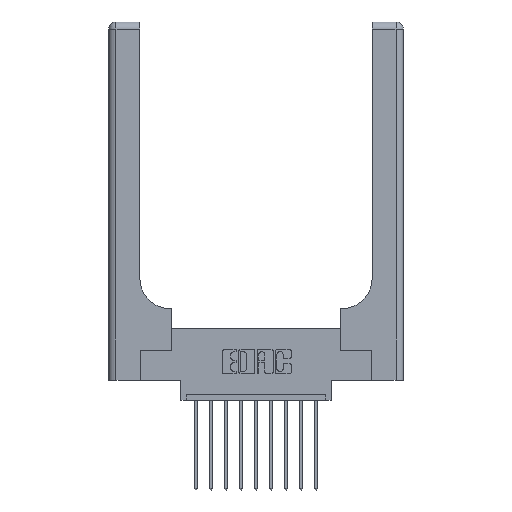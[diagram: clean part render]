
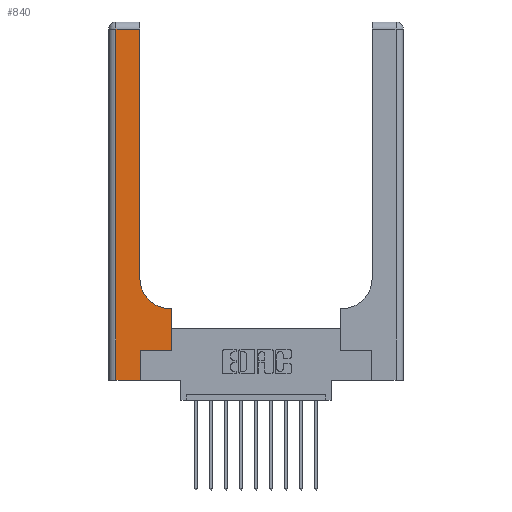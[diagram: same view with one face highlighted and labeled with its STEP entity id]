
A CAD part, top view. The second image highlights one B-rep face of the part: STEP entity #840.
In plain terms, the highlighted planar face has unit normal (0, 0, 1).
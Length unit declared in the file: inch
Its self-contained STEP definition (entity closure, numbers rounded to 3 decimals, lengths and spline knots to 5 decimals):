
#164 = VECTOR ( 'NONE', #4337, 39.37008 ) ;
#223 = EDGE_CURVE ( 'NONE', #14110, #13088, #5973, .T. ) ;
#840 = ADVANCED_FACE ( 'NONE', ( #7039 ), #7645, .F. ) ;
#1093 = VERTEX_POINT ( 'NONE', #11321 ) ;
#1422 = CARTESIAN_POINT ( 'NONE',  ( 0.51, 0.85, 0.37 ) ) ;
#1698 = EDGE_CURVE ( 'NONE', #5517, #12729, #12612, .T. ) ;
#1983 = EDGE_CURVE ( 'NONE', #14137, #7401, #2414, .T. ) ;
#1998 = DIRECTION ( 'NONE',  ( -1., 0., 0. ) ) ;
#2288 = VECTOR ( 'NONE', #9774, 39.37008 ) ;
#2414 = CIRCLE ( 'NONE', #3312, 0.25 ) ;
#2936 = VECTOR ( 'NONE', #14095, 39.37008 ) ;
#3136 = VERTEX_POINT ( 'NONE', #6033 ) ;
#3199 = VECTOR ( 'NONE', #10997, 39.37008 ) ;
#3218 = ORIENTED_EDGE ( 'NONE', *, *, #1983, .T. ) ;
#3287 = CARTESIAN_POINT ( 'NONE',  ( 0.26, 2.94, 0.37 ) ) ;
#3312 = AXIS2_PLACEMENT_3D ( 'NONE', #1422, #7130, #13097 ) ;
#3319 = ORIENTED_EDGE ( 'NONE', *, *, #223, .T. ) ;
#3345 = LINE ( 'NONE', #13888, #164 ) ;
#3554 = CARTESIAN_POINT ( 'NONE',  ( 0.51, 0.6, 0.37 ) ) ;
#3620 = EDGE_LOOP ( 'NONE', ( #14526, #9039, #9863, #4403, #15283, #3319, #12681, #5768, #3218 ) ) ;
#3802 = EDGE_CURVE ( 'NONE', #7401, #14683, #9755, .T. ) ;
#4337 = DIRECTION ( 'NONE',  ( 0., -1., 0. ) ) ;
#4403 = ORIENTED_EDGE ( 'NONE', *, *, #1698, .T. ) ;
#5284 = DIRECTION ( 'NONE',  ( -1., 0., 0. ) ) ;
#5517 = VERTEX_POINT ( 'NONE', #9015 ) ;
#5768 = ORIENTED_EDGE ( 'NONE', *, *, #8043, .T. ) ;
#5973 = LINE ( 'NONE', #12957, #14494 ) ;
#6033 = CARTESIAN_POINT ( 'NONE',  ( 0.528, 0.6, 0.37 ) ) ;
#6101 = CARTESIAN_POINT ( 'NONE',  ( 0.26, 0.85, 0.37 ) ) ;
#6198 = DIRECTION ( 'NONE',  ( 1., 0., 0. ) ) ;
#6939 = DIRECTION ( 'NONE',  ( 0., 1., 0. ) ) ;
#7039 = FACE_OUTER_BOUND ( 'NONE', #3620, .T. ) ;
#7130 = DIRECTION ( 'NONE',  ( 0., 0., -1. ) ) ;
#7401 = VERTEX_POINT ( 'NONE', #6101 ) ;
#7417 = VECTOR ( 'NONE', #6198, 39.37008 ) ;
#7645 = PLANE ( 'NONE',  #10521 ) ;
#7747 = DIRECTION ( 'NONE',  ( 0., 0., -1. ) ) ;
#8011 = LINE ( 'NONE', #10729, #2288 ) ;
#8043 = EDGE_CURVE ( 'NONE', #3136, #14137, #8011, .T. ) ;
#8693 = VECTOR ( 'NONE', #5284, 39.37008 ) ;
#9015 = CARTESIAN_POINT ( 'NONE',  ( 0.06, 0., 0.37 ) ) ;
#9039 = ORIENTED_EDGE ( 'NONE', *, *, #9614, .T. ) ;
#9614 = EDGE_CURVE ( 'NONE', #14683, #1093, #10550, .T. ) ;
#9755 = LINE ( 'NONE', #12920, #2936 ) ;
#9774 = DIRECTION ( 'NONE',  ( -1., 0., 0. ) ) ;
#9863 = ORIENTED_EDGE ( 'NONE', *, *, #15217, .T. ) ;
#10453 = CARTESIAN_POINT ( 'NONE',  ( 0.265, 0., 0.37 ) ) ;
#10521 = AXIS2_PLACEMENT_3D ( 'NONE', #14770, #7747, #1998 ) ;
#10550 = LINE ( 'NONE', #14643, #8693 ) ;
#10729 = CARTESIAN_POINT ( 'NONE',  ( 0.26, 0.6, 0.37 ) ) ;
#10834 = CARTESIAN_POINT ( 'NONE',  ( 0.528, 0.25, 0.37 ) ) ;
#10997 = DIRECTION ( 'NONE',  ( 0., 1., 0. ) ) ;
#11149 = LINE ( 'NONE', #10453, #14080 ) ;
#11321 = CARTESIAN_POINT ( 'NONE',  ( 0.06, 2.94, 0.37 ) ) ;
#11812 = DIRECTION ( 'NONE',  ( 1., 0., 0. ) ) ;
#12027 = CARTESIAN_POINT ( 'NONE',  ( 0.265, 0., 0.37 ) ) ;
#12612 = LINE ( 'NONE', #13285, #7417 ) ;
#12681 = ORIENTED_EDGE ( 'NONE', *, *, #14286, .T. ) ;
#12729 = VERTEX_POINT ( 'NONE', #12027 ) ;
#12920 = CARTESIAN_POINT ( 'NONE',  ( 0.26, 3., 0.37 ) ) ;
#12957 = CARTESIAN_POINT ( 'NONE',  ( 0.265, 0.25, 0.37 ) ) ;
#13088 = VERTEX_POINT ( 'NONE', #15222 ) ;
#13097 = DIRECTION ( 'NONE',  ( 1., 0., 0. ) ) ;
#13285 = CARTESIAN_POINT ( 'NONE',  ( 0., 0., 0.37 ) ) ;
#13748 = LINE ( 'NONE', #10834, #3199 ) ;
#13888 = CARTESIAN_POINT ( 'NONE',  ( 0.06, 3., 0.37 ) ) ;
#14080 = VECTOR ( 'NONE', #6939, 39.37008 ) ;
#14095 = DIRECTION ( 'NONE',  ( 0., 1., 0. ) ) ;
#14110 = VERTEX_POINT ( 'NONE', #15297 ) ;
#14137 = VERTEX_POINT ( 'NONE', #3554 ) ;
#14286 = EDGE_CURVE ( 'NONE', #13088, #3136, #13748, .T. ) ;
#14494 = VECTOR ( 'NONE', #11812, 39.37008 ) ;
#14526 = ORIENTED_EDGE ( 'NONE', *, *, #3802, .T. ) ;
#14643 = CARTESIAN_POINT ( 'NONE',  ( 0., 2.94, 0.37 ) ) ;
#14655 = EDGE_CURVE ( 'NONE', #12729, #14110, #11149, .T. ) ;
#14683 = VERTEX_POINT ( 'NONE', #3287 ) ;
#14770 = CARTESIAN_POINT ( 'NONE',  ( 0., 3., 0.37 ) ) ;
#15217 = EDGE_CURVE ( 'NONE', #1093, #5517, #3345, .T. ) ;
#15222 = CARTESIAN_POINT ( 'NONE',  ( 0.528, 0.25, 0.37 ) ) ;
#15283 = ORIENTED_EDGE ( 'NONE', *, *, #14655, .T. ) ;
#15297 = CARTESIAN_POINT ( 'NONE',  ( 0.265, 0.25, 0.37 ) ) ;
